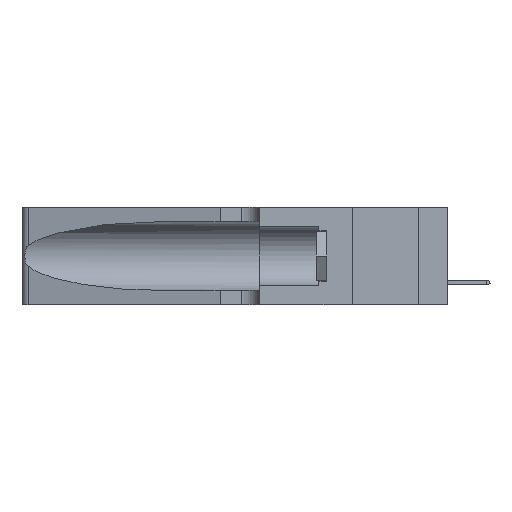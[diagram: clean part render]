
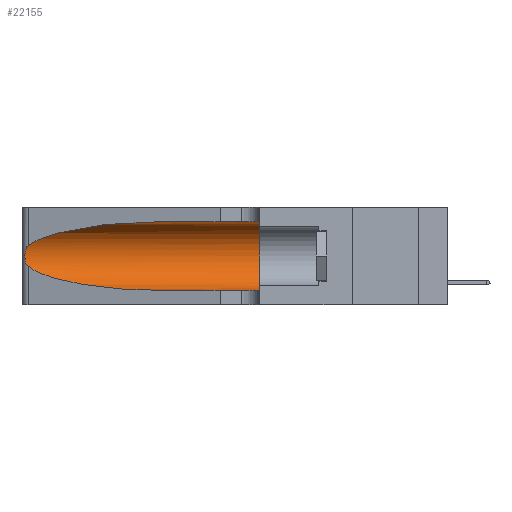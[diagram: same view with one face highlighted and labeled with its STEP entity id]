
A CAD part, left-side view. The second image highlights one B-rep face of the part: STEP entity #22155.
In plain terms, the highlighted cylindrical face has radius 3.308 mm (diameter 6.617 mm), a partial arc.
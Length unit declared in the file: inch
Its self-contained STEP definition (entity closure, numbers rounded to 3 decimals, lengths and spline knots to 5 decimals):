
#754 = DIRECTION ( 'NONE',  ( 0., 1., 0. ) ) ;
#1577 = CIRCLE ( 'NONE', #21522, 0.13025 ) ;
#2148 = CARTESIAN_POINT ( 'NONE',  ( 0.1305, 0.72297, 0.31525 ) ) ;
#2357 = CARTESIAN_POINT ( 'NONE',  ( 0.26018, 1.23835, 0.19895 ) ) ;
#2606 = CARTESIAN_POINT ( 'NONE',  ( 0.18966, 0.96281, 0.31525 ) ) ;
#3005 = LINE ( 'NONE', #5505, #6764 ) ;
#3197 = DIRECTION ( 'NONE',  ( 0., 0., -1. ) ) ;
#3377 = VERTEX_POINT ( 'NONE', #5187 ) ;
#5166 = ORIENTED_EDGE ( 'NONE', *, *, #10389, .T. ) ;
#5187 = CARTESIAN_POINT ( 'NONE',  ( 0.25487, 1.22718, 0.22369 ) ) ;
#5431 = ORIENTED_EDGE ( 'NONE', *, *, #5959, .F. ) ;
#5505 = CARTESIAN_POINT ( 'NONE',  ( 0.1305, 1.61858, 0.31525 ) ) ;
#5816 = CARTESIAN_POINT ( 'NONE',  ( 0.25639, 1.23184, 0.21858 ) ) ;
#5959 = EDGE_CURVE ( 'NONE', #15726, #15105, #1577, .T. ) ;
#6764 = VECTOR ( 'NONE', #13973, 39.37008 ) ;
#7150 = CARTESIAN_POINT ( 'NONE',  ( 0.25487, 1.22718, 0.22369 ) ) ;
#7614 = CARTESIAN_POINT ( 'NONE',  ( 0.25789, 1.23486, 0.15765 ) ) ;
#7755 = CARTESIAN_POINT ( 'NONE',  ( 0.25854, 1.2359, 0.20912 ) ) ;
#7832 = VECTOR ( 'NONE', #14625, 39.37008 ) ;
#8286 = VERTEX_POINT ( 'NONE', #8348 ) ;
#8315 = CARTESIAN_POINT ( 'NONE',  ( 0.1305, 0.35, 0.05475 ) ) ;
#8348 = CARTESIAN_POINT ( 'NONE',  ( 0.1305, 0.72297, 0.05475 ) ) ;
#8364 =( BOUNDED_CURVE ( )  B_SPLINE_CURVE ( 3, ( #20164, #20090, #9622, #21648 ),
 .UNSPECIFIED., .F., .F. ) 
 B_SPLINE_CURVE_WITH_KNOTS ( ( 4, 4 ),
 ( 3.44316, 4.71239 ),
 .UNSPECIFIED. ) 
 CURVE ( )  GEOMETRIC_REPRESENTATION_ITEM ( )  RATIONAL_B_SPLINE_CURVE ( ( 1., 0.87, 0.87, 1. ) ) 
 REPRESENTATION_ITEM ( '' )  );
#8536 = EDGE_CURVE ( 'NONE', #15141, #3377, #16358, .T. ) ;
#8982 = EDGE_CURVE ( 'NONE', #9637, #8286, #8364, .T. ) ;
#9241 = ORIENTED_EDGE ( 'NONE', *, *, #8982, .T. ) ;
#9294 = CARTESIAN_POINT ( 'NONE',  ( 0.25487, 1.22718, 0.14631 ) ) ;
#9484 = CARTESIAN_POINT ( 'NONE',  ( 0.25555, 1.22993, 0.14849 ) ) ;
#9622 = CARTESIAN_POINT ( 'NONE',  ( 0.18966, 0.96281, 0.05475 ) ) ;
#9637 = VERTEX_POINT ( 'NONE', #9294 ) ;
#10389 = EDGE_CURVE ( 'NONE', #3377, #9637, #18738, .T. ) ;
#10697 = ORIENTED_EDGE ( 'NONE', *, *, #18747, .F. ) ;
#10920 = CARTESIAN_POINT ( 'NONE',  ( 0.25639, 1.23186, 0.15144 ) ) ;
#11143 = CARTESIAN_POINT ( 'NONE',  ( 0.26075, 1.23896, 0.178 ) ) ;
#11551 = CARTESIAN_POINT ( 'NONE',  ( 0.1305, 1.61858, 0.05475 ) ) ;
#11715 = FACE_OUTER_BOUND ( 'NONE', #20496, .T. ) ;
#12366 = LINE ( 'NONE', #11551, #7832 ) ;
#12491 = CARTESIAN_POINT ( 'NONE',  ( 0.1305, 0.35, 0.31525 ) ) ;
#12624 = CARTESIAN_POINT ( 'NONE',  ( 0.26017, 1.23833, 0.17102 ) ) ;
#13094 = CARTESIAN_POINT ( 'NONE',  ( 0.1305, 1.61858, 0.185 ) ) ;
#13642 = ORIENTED_EDGE ( 'NONE', *, *, #19514, .T. ) ;
#13973 = DIRECTION ( 'NONE',  ( 0., -1., 0. ) ) ;
#14605 = CARTESIAN_POINT ( 'NONE',  ( 0.1305, 0.35, 0.185 ) ) ;
#14625 = DIRECTION ( 'NONE',  ( 0., -1., 0. ) ) ;
#14683 = CARTESIAN_POINT ( 'NONE',  ( 0.1305, 0.72297, 0.31525 ) ) ;
#15105 = VERTEX_POINT ( 'NONE', #8315 ) ;
#15141 = VERTEX_POINT ( 'NONE', #2148 ) ;
#15726 = VERTEX_POINT ( 'NONE', #12491 ) ;
#15791 = ORIENTED_EDGE ( 'NONE', *, *, #8536, .T. ) ;
#15997 = CARTESIAN_POINT ( 'NONE',  ( 0.25487, 1.22718, 0.14631 ) ) ;
#16154 = CARTESIAN_POINT ( 'NONE',  ( 0.25787, 1.23484, 0.2124 ) ) ;
#16344 = CARTESIAN_POINT ( 'NONE',  ( 0.2373, 1.15595, 0.28018 ) ) ;
#16358 =( BOUNDED_CURVE ( )  B_SPLINE_CURVE ( 3, ( #14683, #2606, #16344, #7150 ),
 .UNSPECIFIED., .F., .F. ) 
 B_SPLINE_CURVE_WITH_KNOTS ( ( 4, 4 ),
 ( 1.5708, 2.84003 ),
 .UNSPECIFIED. ) 
 CURVE ( )  GEOMETRIC_REPRESENTATION_ITEM ( )  RATIONAL_B_SPLINE_CURVE ( ( 1., 0.87, 0.87, 1. ) ) 
 REPRESENTATION_ITEM ( '' )  );
#17850 = CARTESIAN_POINT ( 'NONE',  ( 0.25555, 1.22994, 0.2215 ) ) ;
#18730 = CYLINDRICAL_SURFACE ( 'NONE', #20101, 0.13025 ) ;
#18738 = B_SPLINE_CURVE_WITH_KNOTS ( 'NONE', 3,
 ( #21225, #17850, #5816, #16154, #7755, #2357, #21524, #11143, #12624, #19748, #7614, #10920, #9484, #15997 ),
 .UNSPECIFIED., .F., .F.,
 ( 4, 2, 2, 2, 2, 2, 4 ),
 ( 0., 0.00027, 0.00053, 0.00107, 0.0016, 0.00187, 0.00214 ),
 .UNSPECIFIED. ) ;
#18747 = EDGE_CURVE ( 'NONE', #15141, #15726, #3005, .T. ) ;
#19514 = EDGE_CURVE ( 'NONE', #8286, #15105, #12366, .T. ) ;
#19748 = CARTESIAN_POINT ( 'NONE',  ( 0.25856, 1.23593, 0.16098 ) ) ;
#19993 = DIRECTION ( 'NONE',  ( 0., -1., 0. ) ) ;
#20090 = CARTESIAN_POINT ( 'NONE',  ( 0.2373, 1.15595, 0.08982 ) ) ;
#20101 = AXIS2_PLACEMENT_3D ( 'NONE', #13094, #19993, #3197 ) ;
#20164 = CARTESIAN_POINT ( 'NONE',  ( 0.25487, 1.22718, 0.14631 ) ) ;
#20496 = EDGE_LOOP ( 'NONE', ( #15791, #5166, #9241, #13642, #5431, #10697 ) ) ;
#21225 = CARTESIAN_POINT ( 'NONE',  ( 0.25487, 1.22718, 0.22369 ) ) ;
#21522 = AXIS2_PLACEMENT_3D ( 'NONE', #14605, #754, #21614 ) ;
#21524 = CARTESIAN_POINT ( 'NONE',  ( 0.26075, 1.23896, 0.19203 ) ) ;
#21614 = DIRECTION ( 'NONE',  ( 0., 0., 1. ) ) ;
#21648 = CARTESIAN_POINT ( 'NONE',  ( 0.1305, 0.72297, 0.05475 ) ) ;
#22155 = ADVANCED_FACE ( 'NONE', ( #11715 ), #18730, .F. ) ;
